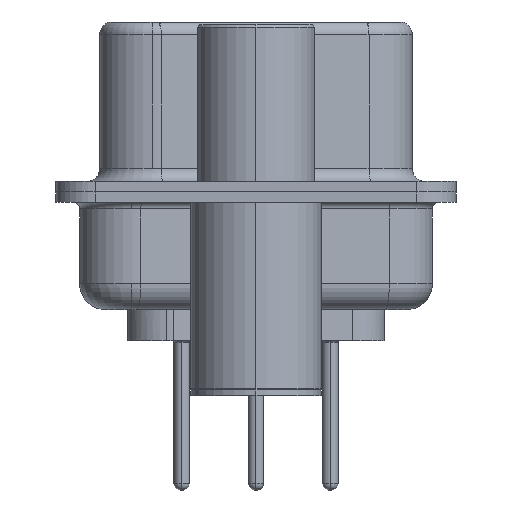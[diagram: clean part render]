
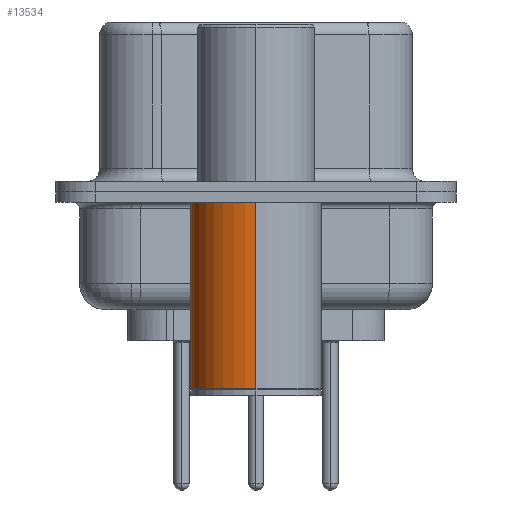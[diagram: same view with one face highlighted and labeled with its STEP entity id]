
A CAD part, left-side view. The second image highlights one B-rep face of the part: STEP entity #13534.
In plain terms, the highlighted cylindrical face has radius 2.5 mm (diameter 5 mm), a partial arc.
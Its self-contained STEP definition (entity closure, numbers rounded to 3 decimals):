
#206 = DIRECTION ( 'NONE',  ( 0., 0., 1. ) ) ;
#458 = DIRECTION ( 'NONE',  ( 0., 0., 1. ) ) ;
#2047 = ORIENTED_EDGE ( 'NONE', *, *, #23110, .T. ) ;
#2142 = ORIENTED_EDGE ( 'NONE', *, *, #26729, .T. ) ;
#2236 = LINE ( 'NONE', #14261, #19501 ) ;
#2743 = ORIENTED_EDGE ( 'NONE', *, *, #28456, .F. ) ;
#3517 = CARTESIAN_POINT ( 'NONE',  ( -2.5, 0., -7.525 ) ) ;
#3717 = CARTESIAN_POINT ( 'NONE',  ( 0., 0., -7.525 ) ) ;
#4310 = VERTEX_POINT ( 'NONE', #3517 ) ;
#4464 = CIRCLE ( 'NONE', #5475, 2.5 ) ;
#5475 = AXIS2_PLACEMENT_3D ( 'NONE', #27951, #30475, #8554 ) ;
#5602 = EDGE_CURVE ( 'NONE', #21893, #25858, #19971, .T. ) ;
#7599 = CYLINDRICAL_SURFACE ( 'NONE', #18062, 2.5 ) ;
#8554 = DIRECTION ( 'NONE',  ( 1., 0., 0. ) ) ;
#11398 = AXIS2_PLACEMENT_3D ( 'NONE', #3717, #22837, #15731 ) ;
#11518 = CARTESIAN_POINT ( 'NONE',  ( 2.5, 0., -0.4 ) ) ;
#12487 = DIRECTION ( 'NONE',  ( 1., 0., 0. ) ) ;
#13534 = ADVANCED_FACE ( 'NONE', ( #14861 ), #7599, .T. ) ;
#14261 = CARTESIAN_POINT ( 'NONE',  ( -2.5, 0., 0.581 ) ) ;
#14861 = FACE_OUTER_BOUND ( 'NONE', #23982, .T. ) ;
#15731 = DIRECTION ( 'NONE',  ( 1., 0., 0. ) ) ;
#18062 = AXIS2_PLACEMENT_3D ( 'NONE', #26846, #458, #12487 ) ;
#19457 = CIRCLE ( 'NONE', #11398, 2.5 ) ;
#19501 = VECTOR ( 'NONE', #28609, 1000. ) ;
#19971 = LINE ( 'NONE', #24234, #27319 ) ;
#20913 = CARTESIAN_POINT ( 'NONE',  ( -2.5, 0., -0.4 ) ) ;
#21834 = VERTEX_POINT ( 'NONE', #20913 ) ;
#21893 = VERTEX_POINT ( 'NONE', #22979 ) ;
#22837 = DIRECTION ( 'NONE',  ( 0., 0., 1. ) ) ;
#22979 = CARTESIAN_POINT ( 'NONE',  ( 2.5, 0., -7.525 ) ) ;
#23110 = EDGE_CURVE ( 'NONE', #21893, #4310, #19457, .T. ) ;
#23982 = EDGE_LOOP ( 'NONE', ( #2047, #2142, #2743, #30875 ) ) ;
#24234 = CARTESIAN_POINT ( 'NONE',  ( 2.5, 0., 0.581 ) ) ;
#25858 = VERTEX_POINT ( 'NONE', #11518 ) ;
#26729 = EDGE_CURVE ( 'NONE', #4310, #21834, #2236, .T. ) ;
#26846 = CARTESIAN_POINT ( 'NONE',  ( 0., 0., 0.581 ) ) ;
#27319 = VECTOR ( 'NONE', #206, 1000. ) ;
#27951 = CARTESIAN_POINT ( 'NONE',  ( 0., 0., -0.4 ) ) ;
#28456 = EDGE_CURVE ( 'NONE', #25858, #21834, #4464, .T. ) ;
#28609 = DIRECTION ( 'NONE',  ( 0., 0., 1. ) ) ;
#30475 = DIRECTION ( 'NONE',  ( 0., 0., 1. ) ) ;
#30875 = ORIENTED_EDGE ( 'NONE', *, *, #5602, .F. ) ;
